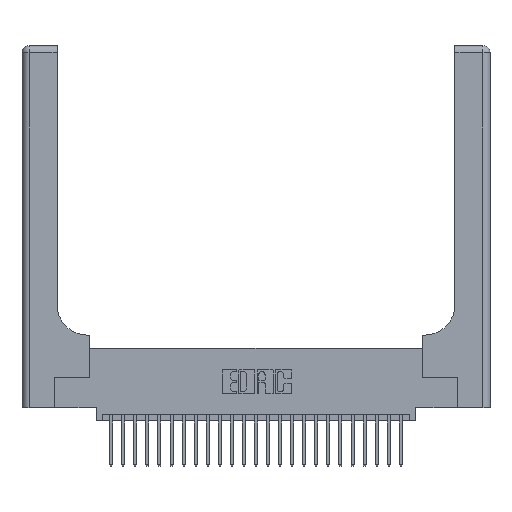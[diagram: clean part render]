
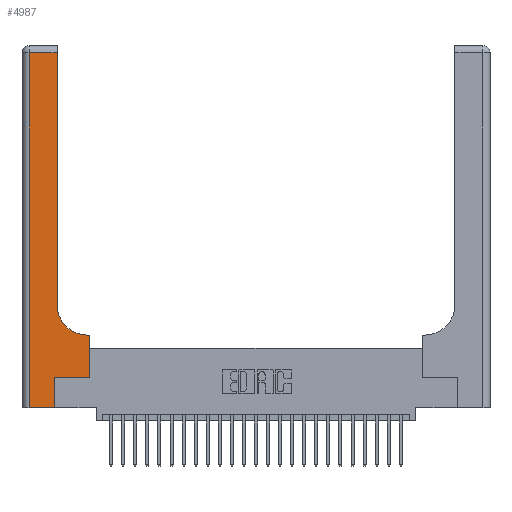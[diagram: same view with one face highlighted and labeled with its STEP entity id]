
A CAD part, top view. The second image highlights one B-rep face of the part: STEP entity #4987.
In plain terms, the highlighted planar face has unit normal (0, 0, 1).
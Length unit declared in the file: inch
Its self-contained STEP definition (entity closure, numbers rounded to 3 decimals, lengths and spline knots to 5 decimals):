
#43 = CARTESIAN_POINT ( 'NONE',  ( 0.269, 0.25, 0.37 ) ) ;
#69 = CARTESIAN_POINT ( 'NONE',  ( 0.5585, 0.6, 0.37 ) ) ;
#812 = VERTEX_POINT ( 'NONE', #19594 ) ;
#909 = LINE ( 'NONE', #11830, #23352 ) ;
#1141 = VECTOR ( 'NONE', #18614, 39.37008 ) ;
#1470 = CARTESIAN_POINT ( 'NONE',  ( 0.5415, 0.85, 0.37 ) ) ;
#1525 = PLANE ( 'NONE',  #19150 ) ;
#2136 = ORIENTED_EDGE ( 'NONE', *, *, #13200, .T. ) ;
#2280 = EDGE_CURVE ( 'NONE', #6709, #8406, #10528, .T. ) ;
#2288 = VECTOR ( 'NONE', #14547, 39.37008 ) ;
#2513 = VERTEX_POINT ( 'NONE', #10514 ) ;
#2736 = EDGE_CURVE ( 'NONE', #15369, #7221, #5472, .T. ) ;
#2860 = DIRECTION ( 'NONE',  ( 0., 1., 0. ) ) ;
#3613 = DIRECTION ( 'NONE',  ( 1., 0., 0. ) ) ;
#3679 = CARTESIAN_POINT ( 'NONE',  ( 0., 3., 0.37 ) ) ;
#3850 = CARTESIAN_POINT ( 'NONE',  ( 0.2915, 3., 0.37 ) ) ;
#4429 = LINE ( 'NONE', #17141, #21240 ) ;
#4433 = VERTEX_POINT ( 'NONE', #22751 ) ;
#4509 = DIRECTION ( 'NONE',  ( 1., 0., 0. ) ) ;
#4828 = VECTOR ( 'NONE', #9117, 39.37008 ) ;
#4873 = CARTESIAN_POINT ( 'NONE',  ( 0.5415, 0.6, 0.37 ) ) ;
#4987 = ADVANCED_FACE ( 'NONE', ( #12058 ), #1525, .F. ) ;
#4995 = CARTESIAN_POINT ( 'NONE',  ( 0.5585, 0.25, 0.37 ) ) ;
#5448 = CARTESIAN_POINT ( 'NONE',  ( 0.06, 2.94, 0.37 ) ) ;
#5472 = LINE ( 'NONE', #17437, #6133 ) ;
#5784 = DIRECTION ( 'NONE',  ( 0., 0., -1. ) ) ;
#6133 = VECTOR ( 'NONE', #23621, 39.37008 ) ;
#6189 = LINE ( 'NONE', #17091, #16772 ) ;
#6709 = VERTEX_POINT ( 'NONE', #69 ) ;
#7221 = VERTEX_POINT ( 'NONE', #43 ) ;
#8406 = VERTEX_POINT ( 'NONE', #4873 ) ;
#8911 = ORIENTED_EDGE ( 'NONE', *, *, #25171, .T. ) ;
#8992 = ORIENTED_EDGE ( 'NONE', *, *, #2280, .T. ) ;
#9117 = DIRECTION ( 'NONE',  ( -1., 0., 0. ) ) ;
#9212 = EDGE_CURVE ( 'NONE', #4433, #12960, #909, .T. ) ;
#9302 = LINE ( 'NONE', #10255, #2288 ) ;
#9599 = CARTESIAN_POINT ( 'NONE',  ( 0.2915, 0.85, 0.37 ) ) ;
#9944 = ORIENTED_EDGE ( 'NONE', *, *, #20498, .T. ) ;
#9959 = ORIENTED_EDGE ( 'NONE', *, *, #19416, .T. ) ;
#10255 = CARTESIAN_POINT ( 'NONE',  ( 0., 0., 0.37 ) ) ;
#10514 = CARTESIAN_POINT ( 'NONE',  ( 0.5585, 0.25, 0.37 ) ) ;
#10528 = LINE ( 'NONE', #23718, #4828 ) ;
#11830 = CARTESIAN_POINT ( 'NONE',  ( 0., 2.94, 0.37 ) ) ;
#12058 = FACE_OUTER_BOUND ( 'NONE', #13777, .T. ) ;
#12960 = VERTEX_POINT ( 'NONE', #5448 ) ;
#13118 = LINE ( 'NONE', #3850, #1141 ) ;
#13200 = EDGE_CURVE ( 'NONE', #7221, #2513, #4429, .T. ) ;
#13777 = EDGE_LOOP ( 'NONE', ( #9944, #21604, #15449, #14708, #16777, #2136, #9959, #8992, #8911 ) ) ;
#13890 = CIRCLE ( 'NONE', #25082, 0.25 ) ;
#13955 = CARTESIAN_POINT ( 'NONE',  ( 0.269, 0., 0.37 ) ) ;
#14512 = EDGE_CURVE ( 'NONE', #12960, #812, #6189, .T. ) ;
#14547 = DIRECTION ( 'NONE',  ( 1., 0., 0. ) ) ;
#14708 = ORIENTED_EDGE ( 'NONE', *, *, #19070, .T. ) ;
#14983 = DIRECTION ( 'NONE',  ( 0., -1., 0. ) ) ;
#15369 = VERTEX_POINT ( 'NONE', #13955 ) ;
#15449 = ORIENTED_EDGE ( 'NONE', *, *, #14512, .T. ) ;
#16265 = DIRECTION ( 'NONE',  ( 0., 0., -1. ) ) ;
#16772 = VECTOR ( 'NONE', #14983, 39.37008 ) ;
#16777 = ORIENTED_EDGE ( 'NONE', *, *, #2736, .T. ) ;
#17091 = CARTESIAN_POINT ( 'NONE',  ( 0.06, 3., 0.37 ) ) ;
#17141 = CARTESIAN_POINT ( 'NONE',  ( 0.269, 0.25, 0.37 ) ) ;
#17437 = CARTESIAN_POINT ( 'NONE',  ( 0.269, 0., 0.37 ) ) ;
#18614 = DIRECTION ( 'NONE',  ( 0., 1., 0. ) ) ;
#19070 = EDGE_CURVE ( 'NONE', #812, #15369, #9302, .T. ) ;
#19150 = AXIS2_PLACEMENT_3D ( 'NONE', #3679, #5784, #20561 ) ;
#19416 = EDGE_CURVE ( 'NONE', #2513, #6709, #26941, .T. ) ;
#19594 = CARTESIAN_POINT ( 'NONE',  ( 0.06, 0., 0.37 ) ) ;
#20498 = EDGE_CURVE ( 'NONE', #21031, #4433, #13118, .T. ) ;
#20561 = DIRECTION ( 'NONE',  ( -1., 0., 0. ) ) ;
#21031 = VERTEX_POINT ( 'NONE', #9599 ) ;
#21240 = VECTOR ( 'NONE', #4509, 39.37008 ) ;
#21453 = VECTOR ( 'NONE', #2860, 39.37008 ) ;
#21604 = ORIENTED_EDGE ( 'NONE', *, *, #9212, .T. ) ;
#22334 = DIRECTION ( 'NONE',  ( -1., 0., 0. ) ) ;
#22751 = CARTESIAN_POINT ( 'NONE',  ( 0.2915, 2.94, 0.37 ) ) ;
#23352 = VECTOR ( 'NONE', #22334, 39.37008 ) ;
#23621 = DIRECTION ( 'NONE',  ( 0., 1., 0. ) ) ;
#23718 = CARTESIAN_POINT ( 'NONE',  ( 0.2915, 0.6, 0.37 ) ) ;
#25082 = AXIS2_PLACEMENT_3D ( 'NONE', #1470, #16265, #3613 ) ;
#25171 = EDGE_CURVE ( 'NONE', #8406, #21031, #13890, .T. ) ;
#26941 = LINE ( 'NONE', #4995, #21453 ) ;
